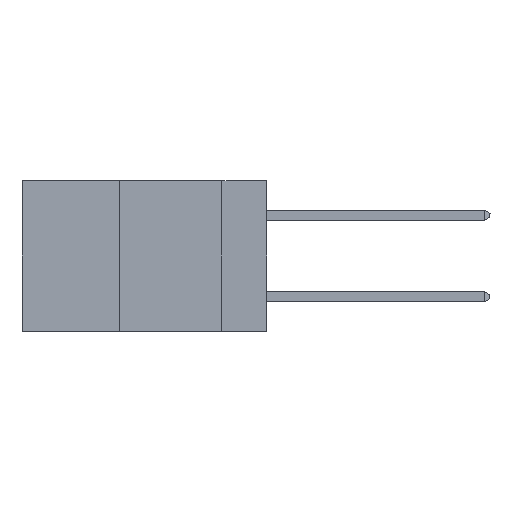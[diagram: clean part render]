
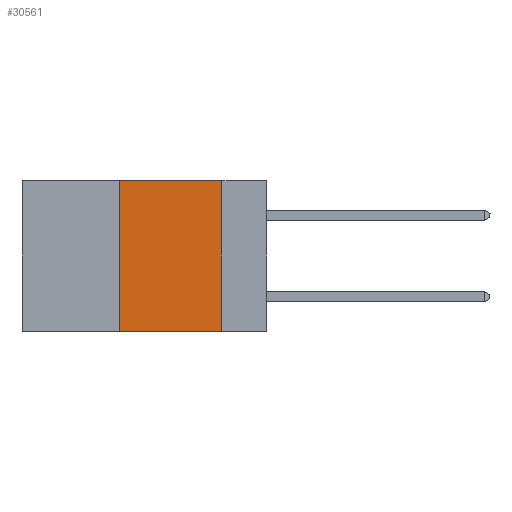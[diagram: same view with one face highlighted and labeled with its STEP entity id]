
A CAD part, left-side view. The second image highlights one B-rep face of the part: STEP entity #30561.
In plain terms, the highlighted planar face has unit normal (-1, 0, 0).
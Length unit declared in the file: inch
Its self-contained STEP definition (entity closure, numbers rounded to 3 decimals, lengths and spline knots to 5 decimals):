
#953 = CARTESIAN_POINT ( 'NONE',  ( 0., 0.11, 0. ) ) ;
#1135 = VERTEX_POINT ( 'NONE', #953 ) ;
#1336 = VECTOR ( 'NONE', #24138, 39.37008 ) ;
#2161 = CARTESIAN_POINT ( 'NONE',  ( 0., 0.11, 0. ) ) ;
#2410 = ORIENTED_EDGE ( 'NONE', *, *, #24273, .F. ) ;
#2529 = ORIENTED_EDGE ( 'NONE', *, *, #35319, .F. ) ;
#3176 = VERTEX_POINT ( 'NONE', #16691 ) ;
#6755 = PLANE ( 'NONE',  #27944 ) ;
#7098 = CARTESIAN_POINT ( 'NONE',  ( 0., 0.6, 0. ) ) ;
#7318 = LINE ( 'NONE', #24571, #23907 ) ;
#7337 = VECTOR ( 'NONE', #18871, 39.37008 ) ;
#7691 = CARTESIAN_POINT ( 'NONE',  ( 0., 0.11, -0.37 ) ) ;
#8484 = CARTESIAN_POINT ( 'NONE',  ( 0., 0.6, 0. ) ) ;
#9447 = DIRECTION ( 'NONE',  ( 0., 0., -1. ) ) ;
#9796 = DIRECTION ( 'NONE',  ( 1., 0., 0. ) ) ;
#10073 = ORIENTED_EDGE ( 'NONE', *, *, #30273, .T. ) ;
#10130 = CARTESIAN_POINT ( 'NONE',  ( 0., 0.36, 0. ) ) ;
#13768 = VECTOR ( 'NONE', #19270, 39.37008 ) ;
#16691 = CARTESIAN_POINT ( 'NONE',  ( 0., 0.36, -0.37 ) ) ;
#17718 = FACE_OUTER_BOUND ( 'NONE', #19358, .T. ) ;
#18871 = DIRECTION ( 'NONE',  ( 0., 0., -1. ) ) ;
#19065 = VERTEX_POINT ( 'NONE', #19670 ) ;
#19270 = DIRECTION ( 'NONE',  ( 0., -1., 0. ) ) ;
#19358 = EDGE_LOOP ( 'NONE', ( #31038, #2529, #2410, #10073 ) ) ;
#19670 = CARTESIAN_POINT ( 'NONE',  ( 0., 0.36, 0. ) ) ;
#21603 = EDGE_CURVE ( 'NONE', #1135, #23520, #29631, .T. ) ;
#22321 = LINE ( 'NONE', #8484, #13768 ) ;
#23520 = VERTEX_POINT ( 'NONE', #7691 ) ;
#23907 = VECTOR ( 'NONE', #29315, 39.37008 ) ;
#24138 = DIRECTION ( 'NONE',  ( 0., 0., 1. ) ) ;
#24273 = EDGE_CURVE ( 'NONE', #3176, #19065, #34735, .T. ) ;
#24571 = CARTESIAN_POINT ( 'NONE',  ( 0., 0.6, -0.37 ) ) ;
#27944 = AXIS2_PLACEMENT_3D ( 'NONE', #7098, #9796, #9447 ) ;
#29315 = DIRECTION ( 'NONE',  ( 0., -1., 0. ) ) ;
#29631 = LINE ( 'NONE', #2161, #7337 ) ;
#30273 = EDGE_CURVE ( 'NONE', #3176, #23520, #7318, .T. ) ;
#30561 = ADVANCED_FACE ( 'NONE', ( #17718 ), #6755, .F. ) ;
#31038 = ORIENTED_EDGE ( 'NONE', *, *, #21603, .F. ) ;
#34735 = LINE ( 'NONE', #10130, #1336 ) ;
#35319 = EDGE_CURVE ( 'NONE', #19065, #1135, #22321, .T. ) ;
